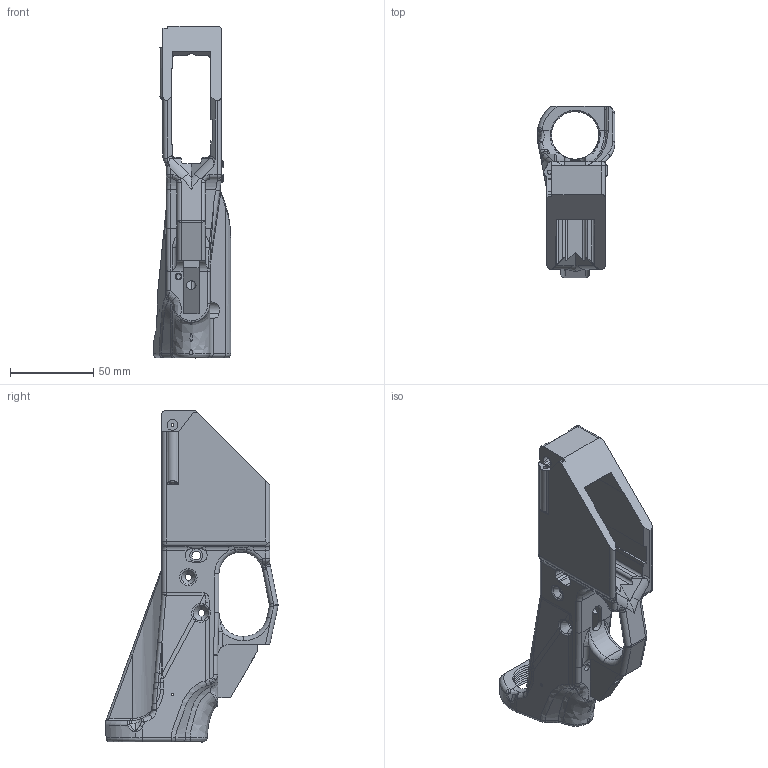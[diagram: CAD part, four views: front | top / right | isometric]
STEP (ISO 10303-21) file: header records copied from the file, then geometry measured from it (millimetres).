
FILE_DESCRIPTION (( 'STEP AP203' ), '1' );
FILE_NAME ('AR Lower V3.0.STEP', '2020-10-02T00:04:43', ( 'Frank' ), ( 'Microsoft' ), 'SwSTEP 2.0', 'SolidWorks 2011', '' );
FILE_SCHEMA (( 'CONFIG_CONTROL_DESIGN' ));
Length unit declared in the file: inch
Products named in the file (1): AR Lower V3.0
Bounding box: 46.72 x 103.45 x 199.48 mm (x, y, z)
Volume: 166525.5 mm3; surface area: 60677.8 mm2
Topology: 1 solids, 1 shells, 753 faces, 2040 edges, 1288 vertices
Faces by surface type: plane 260, cylinder 235, bspline 206, torus 29, sphere 12, cone 11
Entity records: 39360 total; most frequent: CARTESIAN_POINT 22209, ORIENTED_EDGE 4048, DIRECTION 2916, EDGE_CURVE 2024, VERTEX_POINT 1286, VECTOR 978, LINE 978, AXIS2_PLACEMENT_3D 969
